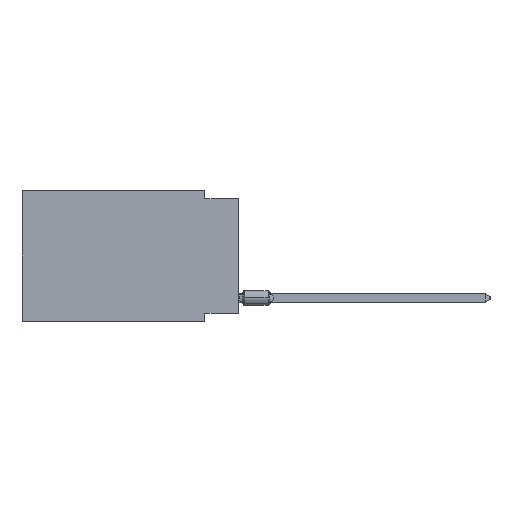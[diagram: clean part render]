
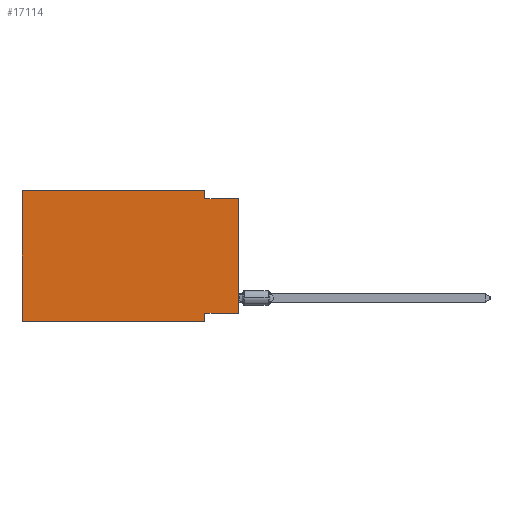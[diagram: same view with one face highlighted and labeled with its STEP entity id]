
A CAD part, left-side view. The second image highlights one B-rep face of the part: STEP entity #17114.
In plain terms, the highlighted planar face has unit normal (-1, 0, 0).
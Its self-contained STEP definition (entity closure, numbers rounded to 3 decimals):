
#3189 = ORIENTED_EDGE ( 'NONE', *, *, #29498, .F. ) ;
#3198 = CARTESIAN_POINT ( 'NONE',  ( 0., 2.54, -9.906 ) ) ;
#3594 = DIRECTION ( 'NONE',  ( 0., -1., 0. ) ) ;
#5965 = CARTESIAN_POINT ( 'NONE',  ( 0., 16.383, 0. ) ) ;
#6290 = ORIENTED_EDGE ( 'NONE', *, *, #60795, .F. ) ;
#6950 = DIRECTION ( 'NONE',  ( 1., 0., 0. ) ) ;
#8071 = VERTEX_POINT ( 'NONE', #12222 ) ;
#10488 = DIRECTION ( 'NONE',  ( 0., 1., 0. ) ) ;
#11042 = VECTOR ( 'NONE', #26435, 1000. ) ;
#11147 = CARTESIAN_POINT ( 'NONE',  ( 0., 0., 0. ) ) ;
#11349 = EDGE_CURVE ( 'NONE', #12811, #8071, #41162, .T. ) ;
#12222 = CARTESIAN_POINT ( 'NONE',  ( 0., 2.54, 0. ) ) ;
#12811 = VERTEX_POINT ( 'NONE', #44656 ) ;
#13640 = LINE ( 'NONE', #28960, #51065 ) ;
#14361 = EDGE_CURVE ( 'NONE', #25865, #12811, #58711, .T. ) ;
#16467 = DIRECTION ( 'NONE',  ( 0., 0., 1. ) ) ;
#17114 = ADVANCED_FACE ( 'NONE', ( #49646 ), #30797, .F. ) ;
#17728 = ORIENTED_EDGE ( 'NONE', *, *, #60350, .T. ) ;
#18233 = EDGE_CURVE ( 'NONE', #54280, #33163, #24952, .T. ) ;
#19179 = VERTEX_POINT ( 'NONE', #19754 ) ;
#19754 = CARTESIAN_POINT ( 'NONE',  ( 0., 2.54, -0.635 ) ) ;
#21995 = VECTOR ( 'NONE', #27886, 1000. ) ;
#22627 = CARTESIAN_POINT ( 'NONE',  ( 0., 16.383, 0. ) ) ;
#24952 = LINE ( 'NONE', #11147, #33574 ) ;
#24961 = VECTOR ( 'NONE', #46687, 1000. ) ;
#25494 = VECTOR ( 'NONE', #10488, 1000. ) ;
#25865 = VERTEX_POINT ( 'NONE', #50702 ) ;
#26072 = CARTESIAN_POINT ( 'NONE',  ( 0., 0., -0.635 ) ) ;
#26435 = DIRECTION ( 'NONE',  ( 0., 0., -1. ) ) ;
#26759 = CARTESIAN_POINT ( 'NONE',  ( 0., 2.54, -9.271 ) ) ;
#27699 = CARTESIAN_POINT ( 'NONE',  ( 0., 0., -9.271 ) ) ;
#27886 = DIRECTION ( 'NONE',  ( 0., -1., 0. ) ) ;
#28960 = CARTESIAN_POINT ( 'NONE',  ( 0., 0., -0.635 ) ) ;
#29498 = EDGE_CURVE ( 'NONE', #54280, #38127, #29924, .T. ) ;
#29924 = LINE ( 'NONE', #44375, #25494 ) ;
#30332 = ORIENTED_EDGE ( 'NONE', *, *, #59632, .F. ) ;
#30797 = PLANE ( 'NONE',  #57460 ) ;
#31447 = LINE ( 'NONE', #3198, #11042 ) ;
#32289 = LINE ( 'NONE', #36681, #21995 ) ;
#33163 = VERTEX_POINT ( 'NONE', #26072 ) ;
#33289 = ORIENTED_EDGE ( 'NONE', *, *, #18233, .T. ) ;
#33574 = VECTOR ( 'NONE', #16467, 1000. ) ;
#35026 = ORIENTED_EDGE ( 'NONE', *, *, #11349, .F. ) ;
#35792 = VERTEX_POINT ( 'NONE', #40799 ) ;
#35800 = DIRECTION ( 'NONE',  ( 0., 0., -1. ) ) ;
#36254 = EDGE_CURVE ( 'NONE', #38127, #35792, #31447, .T. ) ;
#36681 = CARTESIAN_POINT ( 'NONE',  ( 0., 16.383, -9.906 ) ) ;
#38127 = VERTEX_POINT ( 'NONE', #26759 ) ;
#40339 = VECTOR ( 'NONE', #55903, 1000. ) ;
#40799 = CARTESIAN_POINT ( 'NONE',  ( 0., 2.54, -9.906 ) ) ;
#41162 = LINE ( 'NONE', #22627, #40339 ) ;
#44375 = CARTESIAN_POINT ( 'NONE',  ( 0., 0., -9.271 ) ) ;
#44656 = CARTESIAN_POINT ( 'NONE',  ( 0., 16.383, 0. ) ) ;
#46687 = DIRECTION ( 'NONE',  ( 0., 0., -1. ) ) ;
#48482 = ORIENTED_EDGE ( 'NONE', *, *, #14361, .F. ) ;
#49646 = FACE_OUTER_BOUND ( 'NONE', #52671, .T. ) ;
#49945 = CARTESIAN_POINT ( 'NONE',  ( 0., 16.383, 0. ) ) ;
#50382 = VECTOR ( 'NONE', #58399, 1000. ) ;
#50702 = CARTESIAN_POINT ( 'NONE',  ( 0., 16.383, -9.906 ) ) ;
#51065 = VECTOR ( 'NONE', #3594, 1000. ) ;
#52671 = EDGE_LOOP ( 'NONE', ( #33289, #6290, #30332, #35026, #48482, #17728, #59371, #3189 ) ) ;
#54280 = VERTEX_POINT ( 'NONE', #27699 ) ;
#55903 = DIRECTION ( 'NONE',  ( 0., -1., 0. ) ) ;
#56105 = CARTESIAN_POINT ( 'NONE',  ( 0., 2.54, 0. ) ) ;
#56412 = LINE ( 'NONE', #56105, #24961 ) ;
#57460 = AXIS2_PLACEMENT_3D ( 'NONE', #49945, #6950, #35800 ) ;
#58399 = DIRECTION ( 'NONE',  ( 0., 0., 1. ) ) ;
#58711 = LINE ( 'NONE', #5965, #50382 ) ;
#59371 = ORIENTED_EDGE ( 'NONE', *, *, #36254, .F. ) ;
#59632 = EDGE_CURVE ( 'NONE', #8071, #19179, #56412, .T. ) ;
#60350 = EDGE_CURVE ( 'NONE', #25865, #35792, #32289, .T. ) ;
#60795 = EDGE_CURVE ( 'NONE', #19179, #33163, #13640, .T. ) ;
